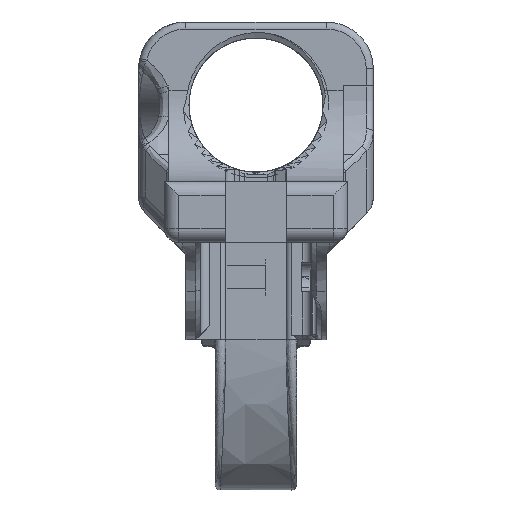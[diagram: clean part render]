
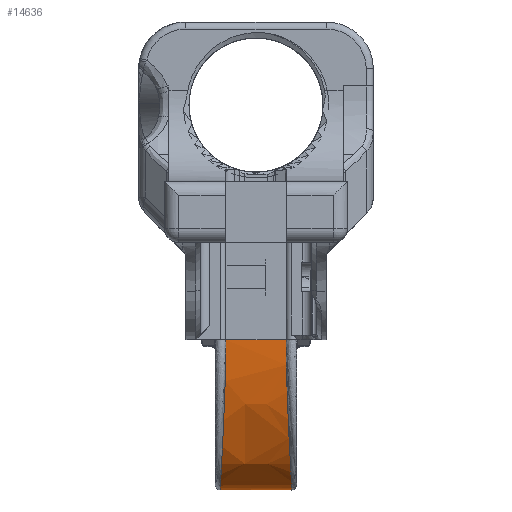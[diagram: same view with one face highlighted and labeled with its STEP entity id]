
A CAD part, left-side view. The second image highlights one B-rep face of the part: STEP entity #14636.
In plain terms, the highlighted free-form (B-spline) face has degree [3, 3] with [4, 4] control points.
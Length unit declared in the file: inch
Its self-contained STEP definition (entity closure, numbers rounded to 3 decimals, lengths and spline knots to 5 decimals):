
#545 = CARTESIAN_POINT ( 'NONE',  ( 0.31264, 0.30113, -3.85823 ) ) ;
#575 = CARTESIAN_POINT ( 'NONE',  ( -0.16815, -0.30113, -3.85823 ) ) ;
#1401 = CARTESIAN_POINT ( 'NONE',  ( -0.38772, -0.25252, -2.59823 ) ) ;
#2830 = CARTESIAN_POINT ( 'NONE',  ( -0.38772, 0.25252, -2.59823 ) ) ;
#3490 = CARTESIAN_POINT ( 'NONE',  ( 0.31264, 0.30113, -3.85823 ) ) ;
#3692 = VECTOR ( 'NONE', #25620, 39.37008 ) ;
#3737 = CARTESIAN_POINT ( 'NONE',  ( 0.31264, 0.30113, -3.85823 ) ) ;
#3913 = CARTESIAN_POINT ( 'NONE',  ( 0.31264, -0.30113, -3.85823 ) ) ;
#4379 = CARTESIAN_POINT ( 'NONE',  ( 0.31264, 0.10038, -3.85823 ) ) ;
#4961 = ORIENTED_EDGE ( 'NONE', *, *, #32077, .T. ) ;
#5017 = ORIENTED_EDGE ( 'NONE', *, *, #15154, .T. ) ;
#5084 = EDGE_CURVE ( 'NONE', #25430, #9833, #13086, .T. ) ;
#5172 = CARTESIAN_POINT ( 'NONE',  ( 0.31264, -0.10038, -3.85823 ) ) ;
#5764 = CARTESIAN_POINT ( 'NONE',  ( -0.38772, -0.25252, -3.07902 ) ) ;
#6083 = CARTESIAN_POINT ( 'NONE',  ( -0.38772, 0.25252, -2.59823 ) ) ;
#6641 = VERTEX_POINT ( 'NONE', #3913 ) ;
#6823 = CARTESIAN_POINT ( 'NONE',  ( -0.38772, 0., -2.59823 ) ) ;
#7447 = CARTESIAN_POINT ( 'NONE',  ( -0.38772, -0.08417, -3.07902 ) ) ;
#7765 = CARTESIAN_POINT ( 'NONE',  ( -0.16815, 0.30113, -3.85823 ) ) ;
#8664 = CARTESIAN_POINT ( 'NONE',  ( -0.38772, 0.25252, -3.07902 ) ) ;
#9833 = VERTEX_POINT ( 'NONE', #545 ) ;
#10735 = LINE ( 'NONE', #6823, #25249 ) ;
#12934 = CARTESIAN_POINT ( 'NONE',  ( 0.31264, -0.30113, -3.85823 ) ) ;
#13086 = B_SPLINE_CURVE_WITH_KNOTS ( 'NONE', 3,
 ( #6083, #8664, #21537, #3490 ),
 .UNSPECIFIED., .F., .F.,
 ( 4, 4 ),
 ( 0., 1. ),
 .UNSPECIFIED. ) ;
#13799 = FACE_OUTER_BOUND ( 'NONE', #15552, .T. ) ;
#14330 = LINE ( 'NONE', #20472, #3692 ) ;
#14636 = ADVANCED_FACE ( 'NONE', ( #13799 ), #18734, .T. ) ;
#14661 = CARTESIAN_POINT ( 'NONE',  ( -0.38772, 0.25252, -2.59823 ) ) ;
#15154 = EDGE_CURVE ( 'NONE', #27882, #25430, #10735, .T. ) ;
#15552 = EDGE_LOOP ( 'NONE', ( #4961, #21736, #5017, #27471 ) ) ;
#15799 = B_SPLINE_CURVE_WITH_KNOTS ( 'NONE', 3,
 ( #18601, #575, #5764, #23773 ),
 .UNSPECIFIED., .F., .F.,
 ( 4, 4 ),
 ( 0., 1. ),
 .UNSPECIFIED. ) ;
#16855 = CARTESIAN_POINT ( 'NONE',  ( -0.38772, -0.25252, -3.07902 ) ) ;
#17691 = CARTESIAN_POINT ( 'NONE',  ( -0.38772, 0.08417, -2.59823 ) ) ;
#18601 = CARTESIAN_POINT ( 'NONE',  ( 0.31264, -0.30113, -3.85823 ) ) ;
#18734 = B_SPLINE_SURFACE_WITH_KNOTS ( 'NONE', 3, 3, ( 
 ( #3737, #7765, #30044, #14661 ),
 ( #4379, #28551, #23091, #17691 ),
 ( #5172, #25431, #7447, #25660 ),
 ( #12934, #27449, #16855, #1401 ) ),
 .UNSPECIFIED., .F., .F., .F.,
 ( 4, 4 ),
 ( 4, 4 ),
 ( 0., 1. ),
 ( 0., 1. ),
 .UNSPECIFIED. ) ;
#20472 = CARTESIAN_POINT ( 'NONE',  ( 0.31264, 0.73097, -3.85823 ) ) ;
#21537 = CARTESIAN_POINT ( 'NONE',  ( -0.16815, 0.30113, -3.85823 ) ) ;
#21736 = ORIENTED_EDGE ( 'NONE', *, *, #25491, .T. ) ;
#22945 = CARTESIAN_POINT ( 'NONE',  ( -0.38772, -0.25252, -2.59823 ) ) ;
#23091 = CARTESIAN_POINT ( 'NONE',  ( -0.38772, 0.08417, -3.07902 ) ) ;
#23773 = CARTESIAN_POINT ( 'NONE',  ( -0.38772, -0.25252, -2.59823 ) ) ;
#25249 = VECTOR ( 'NONE', #32717, 39.37008 ) ;
#25430 = VERTEX_POINT ( 'NONE', #2830 ) ;
#25431 = CARTESIAN_POINT ( 'NONE',  ( -0.16815, -0.10038, -3.85823 ) ) ;
#25491 = EDGE_CURVE ( 'NONE', #6641, #27882, #15799, .T. ) ;
#25620 = DIRECTION ( 'NONE',  ( 0., -1., 0. ) ) ;
#25660 = CARTESIAN_POINT ( 'NONE',  ( -0.38772, -0.08417, -2.59823 ) ) ;
#27449 = CARTESIAN_POINT ( 'NONE',  ( -0.16815, -0.30113, -3.85823 ) ) ;
#27471 = ORIENTED_EDGE ( 'NONE', *, *, #5084, .T. ) ;
#27882 = VERTEX_POINT ( 'NONE', #22945 ) ;
#28551 = CARTESIAN_POINT ( 'NONE',  ( -0.16815, 0.10038, -3.85823 ) ) ;
#30044 = CARTESIAN_POINT ( 'NONE',  ( -0.38772, 0.25252, -3.07902 ) ) ;
#32077 = EDGE_CURVE ( 'NONE', #9833, #6641, #14330, .T. ) ;
#32717 = DIRECTION ( 'NONE',  ( 0., 1., 0. ) ) ;
